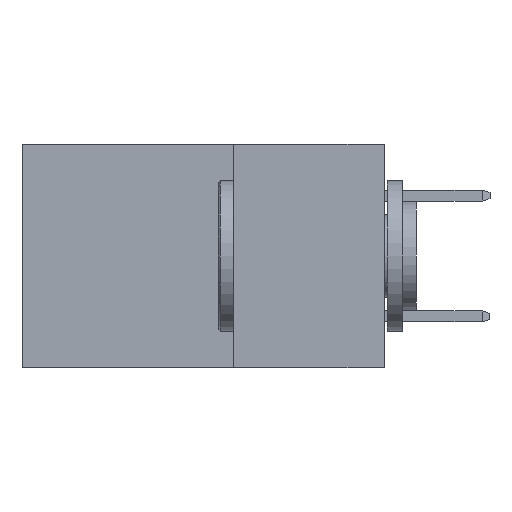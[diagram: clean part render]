
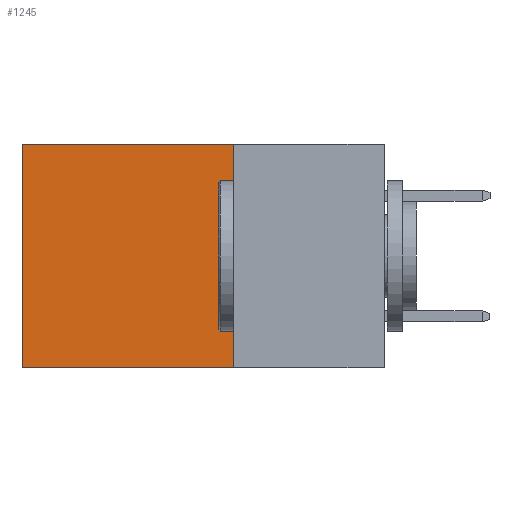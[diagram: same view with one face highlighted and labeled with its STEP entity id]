
A CAD part, left-side view. The second image highlights one B-rep face of the part: STEP entity #1245.
In plain terms, the highlighted planar face has unit normal (-1, 0, 0).
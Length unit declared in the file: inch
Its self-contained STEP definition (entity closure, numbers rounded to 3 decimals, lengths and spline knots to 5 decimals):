
#450 = CARTESIAN_POINT ( 'NONE',  ( 0.298, 0.6, 0. ) ) ;
#848 = LINE ( 'NONE', #7089, #18629 ) ;
#888 = CARTESIAN_POINT ( 'NONE',  ( 0.298, 0.6, -0.37 ) ) ;
#1122 = CARTESIAN_POINT ( 'NONE',  ( 0.298, 0.6, 0. ) ) ;
#1245 = ADVANCED_FACE ( 'NONE', ( #14525 ), #2041, .F. ) ;
#1247 = VERTEX_POINT ( 'NONE', #888 ) ;
#1288 = CARTESIAN_POINT ( 'NONE',  ( 0.298, 0.25, 0. ) ) ;
#2041 = PLANE ( 'NONE',  #2358 ) ;
#2358 = AXIS2_PLACEMENT_3D ( 'NONE', #1288, #4595, #3705 ) ;
#3705 = DIRECTION ( 'NONE',  ( 0., 0., -1. ) ) ;
#4595 = DIRECTION ( 'NONE',  ( 1., 0., 0. ) ) ;
#6737 = DIRECTION ( 'NONE',  ( 0., 1., 0. ) ) ;
#6977 = ORIENTED_EDGE ( 'NONE', *, *, #21456, .T. ) ;
#7089 = CARTESIAN_POINT ( 'NONE',  ( 0.298, 0.25, -0.37 ) ) ;
#7267 = LINE ( 'NONE', #18168, #12277 ) ;
#7334 = VERTEX_POINT ( 'NONE', #12260 ) ;
#7665 = LINE ( 'NONE', #450, #17700 ) ;
#9253 = VERTEX_POINT ( 'NONE', #1122 ) ;
#9672 = ORIENTED_EDGE ( 'NONE', *, *, #15351, .T. ) ;
#11680 = CARTESIAN_POINT ( 'NONE',  ( 0.298, 0.25, 0. ) ) ;
#11799 = EDGE_CURVE ( 'NONE', #15232, #7334, #7267, .T. ) ;
#12260 = CARTESIAN_POINT ( 'NONE',  ( 0.298, 0.25, -0.37 ) ) ;
#12277 = VECTOR ( 'NONE', #18249, 39.37008 ) ;
#14155 = EDGE_CURVE ( 'NONE', #7334, #1247, #848, .T. ) ;
#14525 = FACE_OUTER_BOUND ( 'NONE', #22514, .T. ) ;
#14934 = ORIENTED_EDGE ( 'NONE', *, *, #11799, .F. ) ;
#15232 = VERTEX_POINT ( 'NONE', #11680 ) ;
#15351 = EDGE_CURVE ( 'NONE', #9253, #1247, #7665, .T. ) ;
#16660 = DIRECTION ( 'NONE',  ( 0., 1., 0. ) ) ;
#17700 = VECTOR ( 'NONE', #21314, 39.37008 ) ;
#18168 = CARTESIAN_POINT ( 'NONE',  ( 0.298, 0.25, 0. ) ) ;
#18249 = DIRECTION ( 'NONE',  ( 0., 0., -1. ) ) ;
#18569 = LINE ( 'NONE', #23873, #22818 ) ;
#18629 = VECTOR ( 'NONE', #6737, 39.37008 ) ;
#18817 = ORIENTED_EDGE ( 'NONE', *, *, #14155, .F. ) ;
#21314 = DIRECTION ( 'NONE',  ( 0., 0., -1. ) ) ;
#21456 = EDGE_CURVE ( 'NONE', #15232, #9253, #18569, .T. ) ;
#22514 = EDGE_LOOP ( 'NONE', ( #9672, #18817, #14934, #6977 ) ) ;
#22818 = VECTOR ( 'NONE', #16660, 39.37008 ) ;
#23873 = CARTESIAN_POINT ( 'NONE',  ( 0.298, 0.25, 0. ) ) ;
